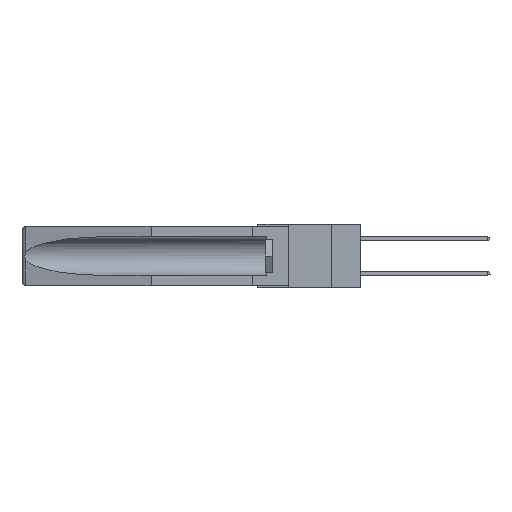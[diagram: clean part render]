
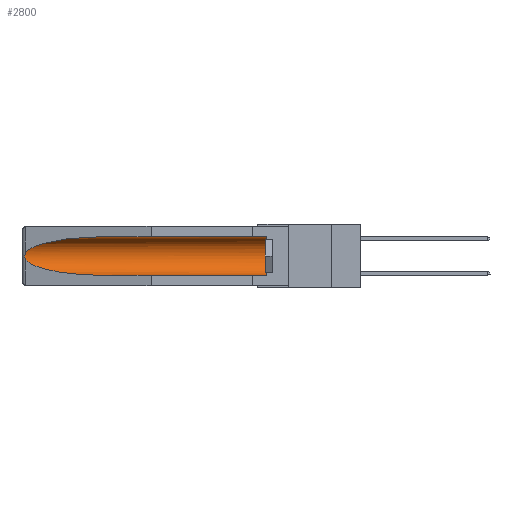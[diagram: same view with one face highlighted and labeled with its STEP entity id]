
A CAD part, left-side view. The second image highlights one B-rep face of the part: STEP entity #2800.
In plain terms, the highlighted cylindrical face has radius 2.857 mm (diameter 5.715 mm), a partial arc.
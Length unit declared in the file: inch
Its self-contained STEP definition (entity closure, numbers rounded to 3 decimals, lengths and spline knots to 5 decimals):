
#98 = EDGE_CURVE ( 'NONE', #22337, #4815, #23288, .T. ) ;
#237 = CARTESIAN_POINT ( 'NONE',  ( 0.26597, 1.5296, -0.19026 ) ) ;
#263 = EDGE_CURVE ( 'NONE', #9077, #22337, #11384, .T. ) ;
#744 = ORIENTED_EDGE ( 'NONE', *, *, #11237, .F. ) ;
#1615 = CARTESIAN_POINT ( 'NONE',  ( 0.26537, 1.52718, -0.19328 ) ) ;
#1911 =( BOUNDED_CURVE ( )  B_SPLINE_CURVE ( 3, ( #1615, #16658, #3543, #12938 ),
 .UNSPECIFIED., .F., .F. ) 
 B_SPLINE_CURVE_WITH_KNOTS ( ( 4, 4 ),
 ( 0.1948, 1.5708 ),
 .UNSPECIFIED. ) 
 CURVE ( )  GEOMETRIC_REPRESENTATION_ITEM ( )  RATIONAL_B_SPLINE_CURVE ( ( 1., 0.848, 0.848, 1. ) ) 
 REPRESENTATION_ITEM ( '' )  );
#2173 = CARTESIAN_POINT ( 'NONE',  ( 0.155, -0.30754, -0.284 ) ) ;
#2430 = CARTESIAN_POINT ( 'NONE',  ( 0.155, 0.126, -0.1715 ) ) ;
#2495 = CARTESIAN_POINT ( 'NONE',  ( 0.26537, 1.52718, -0.14972 ) ) ;
#2512 = CARTESIAN_POINT ( 'NONE',  ( 0.155, 0.126, -0.284 ) ) ;
#2800 = ADVANCED_FACE ( 'NONE', ( #16515 ), #18928, .F. ) ;
#3543 = CARTESIAN_POINT ( 'NONE',  ( 0.21114, 1.30732, -0.284 ) ) ;
#4406 = CARTESIAN_POINT ( 'NONE',  ( 0.26654, 1.53092, -0.15636 ) ) ;
#4815 = VERTEX_POINT ( 'NONE', #15239 ) ;
#6450 = VERTEX_POINT ( 'NONE', #11109 ) ;
#6958 = AXIS2_PLACEMENT_3D ( 'NONE', #2430, #19385, #11916 ) ;
#7149 = ORIENTED_EDGE ( 'NONE', *, *, #98, .T. ) ;
#7484 = ORIENTED_EDGE ( 'NONE', *, *, #19432, .T. ) ;
#8114 = DIRECTION ( 'NONE',  ( 0., 0., 1. ) ) ;
#8881 = CARTESIAN_POINT ( 'NONE',  ( 0.21114, 1.30732, -0.059 ) ) ;
#9077 = VERTEX_POINT ( 'NONE', #2512 ) ;
#9842 = CARTESIAN_POINT ( 'NONE',  ( 0.26597, 1.52961, -0.15275 ) ) ;
#11109 = CARTESIAN_POINT ( 'NONE',  ( 0.26537, 1.52718, -0.14972 ) ) ;
#11167 = VECTOR ( 'NONE', #17309, 39.37008 ) ;
#11237 = EDGE_CURVE ( 'NONE', #9077, #18060, #20684, .T. ) ;
#11384 = CIRCLE ( 'NONE', #6958, 0.1125 ) ;
#11916 = DIRECTION ( 'NONE',  ( 0., 0., 1. ) ) ;
#12753 = CARTESIAN_POINT ( 'NONE',  ( 0.26537, 1.52718, -0.19328 ) ) ;
#12938 = CARTESIAN_POINT ( 'NONE',  ( 0.155, 1.07973, -0.284 ) ) ;
#13720 = CARTESIAN_POINT ( 'NONE',  ( 0.26537, 1.52718, -0.19328 ) ) ;
#13802 = CARTESIAN_POINT ( 'NONE',  ( 0.2673, 1.53269, -0.17917 ) ) ;
#15239 = CARTESIAN_POINT ( 'NONE',  ( 0.155, 1.07973, -0.059 ) ) ;
#15628 =( BOUNDED_CURVE ( )  B_SPLINE_CURVE ( 3, ( #20182, #8881, #18502, #20274 ),
 .UNSPECIFIED., .F., .F. ) 
 B_SPLINE_CURVE_WITH_KNOTS ( ( 4, 4 ),
 ( 4.71239, 6.08839 ),
 .UNSPECIFIED. ) 
 CURVE ( )  GEOMETRIC_REPRESENTATION_ITEM ( )  RATIONAL_B_SPLINE_CURVE ( ( 1., 0.848, 0.848, 1. ) ) 
 REPRESENTATION_ITEM ( '' )  );
#15676 = CARTESIAN_POINT ( 'NONE',  ( 0.155, -0.30754, -0.1715 ) ) ;
#15689 = ORIENTED_EDGE ( 'NONE', *, *, #263, .T. ) ;
#15710 = CARTESIAN_POINT ( 'NONE',  ( 0.26655, 1.53094, -0.18657 ) ) ;
#15792 = CARTESIAN_POINT ( 'NONE',  ( 0.2673, 1.5327, -0.16383 ) ) ;
#15862 = ORIENTED_EDGE ( 'NONE', *, *, #19895, .T. ) ;
#16441 = AXIS2_PLACEMENT_3D ( 'NONE', #15676, #18893, #8114 ) ;
#16515 = FACE_OUTER_BOUND ( 'NONE', #19095, .T. ) ;
#16658 = CARTESIAN_POINT ( 'NONE',  ( 0.25451, 1.48313, -0.24835 ) ) ;
#16704 = DIRECTION ( 'NONE',  ( 0., 1., 0. ) ) ;
#16767 = VERTEX_POINT ( 'NONE', #12753 ) ;
#17309 = DIRECTION ( 'NONE',  ( 0., 1., 0. ) ) ;
#17760 = CARTESIAN_POINT ( 'NONE',  ( 0.155, 1.07973, -0.284 ) ) ;
#18060 = VERTEX_POINT ( 'NONE', #17760 ) ;
#18502 = CARTESIAN_POINT ( 'NONE',  ( 0.25451, 1.48313, -0.09465 ) ) ;
#18544 = EDGE_CURVE ( 'NONE', #6450, #16767, #21142, .T. ) ;
#18893 = DIRECTION ( 'NONE',  ( 0., 1., 0. ) ) ;
#18928 = CYLINDRICAL_SURFACE ( 'NONE', #16441, 0.1125 ) ;
#19095 = EDGE_LOOP ( 'NONE', ( #7484, #20987, #15862, #744, #15689, #7149 ) ) ;
#19283 = CARTESIAN_POINT ( 'NONE',  ( 0.2675, 1.53308, -0.17534 ) ) ;
#19385 = DIRECTION ( 'NONE',  ( 0., -1., 0. ) ) ;
#19432 = EDGE_CURVE ( 'NONE', #4815, #6450, #15628, .T. ) ;
#19895 = EDGE_CURVE ( 'NONE', #16767, #18060, #1911, .T. ) ;
#20182 = CARTESIAN_POINT ( 'NONE',  ( 0.155, 1.07973, -0.059 ) ) ;
#20274 = CARTESIAN_POINT ( 'NONE',  ( 0.26537, 1.52718, -0.14972 ) ) ;
#20684 = LINE ( 'NONE', #2173, #11167 ) ;
#20732 = CARTESIAN_POINT ( 'NONE',  ( 0.155, -0.30754, -0.059 ) ) ;
#20987 = ORIENTED_EDGE ( 'NONE', *, *, #18544, .T. ) ;
#21142 = B_SPLINE_CURVE_WITH_KNOTS ( 'NONE', 3,
 ( #2495, #9842, #4406, #15792, #21304, #19283, #13802, #15710, #237, #13720 ),
 .UNSPECIFIED., .F., .F.,
 ( 4, 2, 2, 2, 4 ),
 ( 0., 0.00029, 0.00058, 0.00087, 0.00117 ),
 .UNSPECIFIED. ) ;
#21304 = CARTESIAN_POINT ( 'NONE',  ( 0.2675, 1.53308, -0.16763 ) ) ;
#21861 = CARTESIAN_POINT ( 'NONE',  ( 0.155, 0.126, -0.059 ) ) ;
#22337 = VERTEX_POINT ( 'NONE', #21861 ) ;
#23257 = VECTOR ( 'NONE', #16704, 39.37008 ) ;
#23288 = LINE ( 'NONE', #20732, #23257 ) ;
